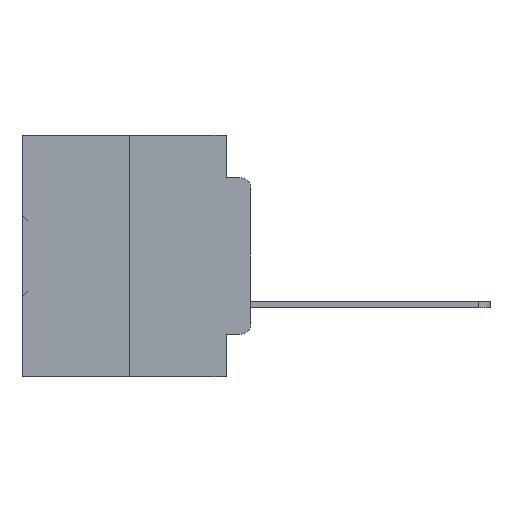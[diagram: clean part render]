
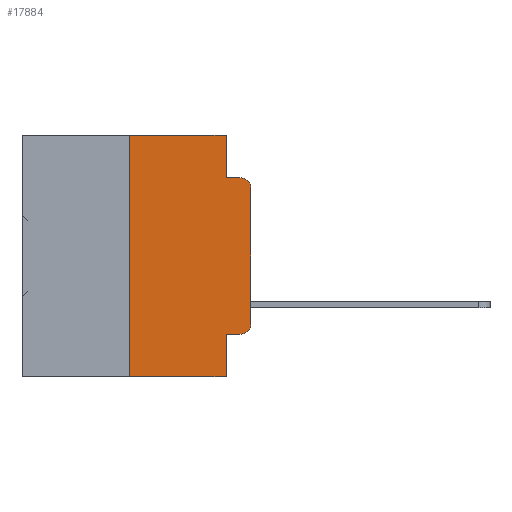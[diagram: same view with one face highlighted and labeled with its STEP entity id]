
A CAD part, left-side view. The second image highlights one B-rep face of the part: STEP entity #17884.
In plain terms, the highlighted planar face has unit normal (-1, 0, 0).
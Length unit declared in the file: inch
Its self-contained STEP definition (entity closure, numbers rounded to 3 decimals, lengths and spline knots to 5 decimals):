
#5 = VERTEX_POINT ( 'NONE', #21967 ) ;
#500 = LINE ( 'NONE', #32016, #10309 ) ;
#594 = DIRECTION ( 'NONE',  ( 0., 0., -1. ) ) ;
#1216 = VERTEX_POINT ( 'NONE', #17893 ) ;
#2350 = DIRECTION ( 'NONE',  ( 0., 0., 1. ) ) ;
#2479 = CARTESIAN_POINT ( 'NONE',  ( 0., 0., 0. ) ) ;
#2881 = VERTEX_POINT ( 'NONE', #8813 ) ;
#3115 = CARTESIAN_POINT ( 'NONE',  ( 0., 0.051, -0.4115 ) ) ;
#3571 = EDGE_CURVE ( 'NONE', #1216, #13545, #20592, .T. ) ;
#4663 = VERTEX_POINT ( 'NONE', #7876 ) ;
#5486 = ORIENTED_EDGE ( 'NONE', *, *, #15837, .T. ) ;
#6073 = VERTEX_POINT ( 'NONE', #37054 ) ;
#7161 = DIRECTION ( 'NONE',  ( 0., -1., 0. ) ) ;
#7540 = VECTOR ( 'NONE', #7161, 39.37008 ) ;
#7876 = CARTESIAN_POINT ( 'NONE',  ( 0., 0.051, -0.4115 ) ) ;
#8208 = DIRECTION ( 'NONE',  ( -1., 0., 0. ) ) ;
#8439 = DIRECTION ( 'NONE',  ( 0., 0., -1. ) ) ;
#8753 = VECTOR ( 'NONE', #594, 39.37008 ) ;
#8813 = CARTESIAN_POINT ( 'NONE',  ( 0., 0., -0.1085 ) ) ;
#8851 = CARTESIAN_POINT ( 'NONE',  ( 0., 0.02, -0.0885 ) ) ;
#8974 = DIRECTION ( 'NONE',  ( 0., -1., 0. ) ) ;
#9942 = VERTEX_POINT ( 'NONE', #20865 ) ;
#10309 = VECTOR ( 'NONE', #2350, 39.37008 ) ;
#10937 = EDGE_CURVE ( 'NONE', #20522, #1216, #16654, .T. ) ;
#11811 = VECTOR ( 'NONE', #24038, 39.37008 ) ;
#11969 = CIRCLE ( 'NONE', #26643, 0.02 ) ;
#13545 = VERTEX_POINT ( 'NONE', #8851 ) ;
#13551 = ORIENTED_EDGE ( 'NONE', *, *, #27134, .T. ) ;
#13850 = VERTEX_POINT ( 'NONE', #27677 ) ;
#15076 = CARTESIAN_POINT ( 'NONE',  ( 0., 0.051, 0. ) ) ;
#15723 = FACE_OUTER_BOUND ( 'NONE', #20264, .T. ) ;
#15837 = EDGE_CURVE ( 'NONE', #2881, #13545, #23999, .T. ) ;
#16018 = EDGE_CURVE ( 'NONE', #4663, #13850, #22566, .T. ) ;
#16654 = LINE ( 'NONE', #15076, #8753 ) ;
#17280 = DIRECTION ( 'NONE',  ( 0., 0., -1. ) ) ;
#17533 = LINE ( 'NONE', #26480, #19832 ) ;
#17884 = ADVANCED_FACE ( 'NONE', ( #15723 ), #35741, .F. ) ;
#17893 = CARTESIAN_POINT ( 'NONE',  ( 0., 0.051, -0.0885 ) ) ;
#19577 = ORIENTED_EDGE ( 'NONE', *, *, #16018, .T. ) ;
#19580 = VECTOR ( 'NONE', #20387, 39.37008 ) ;
#19832 = VECTOR ( 'NONE', #38354, 39.37008 ) ;
#19879 = CARTESIAN_POINT ( 'NONE',  ( 0., 0.02, -0.1085 ) ) ;
#20264 = EDGE_LOOP ( 'NONE', ( #27357, #5486, #26753, #24312, #37018, #27078, #20570, #24830, #19577, #13551 ) ) ;
#20350 = VECTOR ( 'NONE', #8439, 39.37008 ) ;
#20387 = DIRECTION ( 'NONE',  ( 0., 0., 1. ) ) ;
#20522 = VERTEX_POINT ( 'NONE', #36520 ) ;
#20570 = ORIENTED_EDGE ( 'NONE', *, *, #32765, .T. ) ;
#20592 = LINE ( 'NONE', #26526, #11811 ) ;
#20865 = CARTESIAN_POINT ( 'NONE',  ( 0., 0., -0.3915 ) ) ;
#21633 = VECTOR ( 'NONE', #8974, 39.37008 ) ;
#21931 = EDGE_CURVE ( 'NONE', #9942, #2881, #30766, .T. ) ;
#21935 = DIRECTION ( 'NONE',  ( -1., 0., 0. ) ) ;
#21967 = CARTESIAN_POINT ( 'NONE',  ( 0., 0.25, -0.5 ) ) ;
#22069 = CARTESIAN_POINT ( 'NONE',  ( 0., 0.02, -0.3915 ) ) ;
#22077 = CARTESIAN_POINT ( 'NONE',  ( 0., 0.473, 0. ) ) ;
#22566 = LINE ( 'NONE', #3115, #21633 ) ;
#23635 = CARTESIAN_POINT ( 'NONE',  ( 0., 0.473, 0. ) ) ;
#23999 = CIRCLE ( 'NONE', #29081, 0.02 ) ;
#24038 = DIRECTION ( 'NONE',  ( 0., -1., 0. ) ) ;
#24096 = LINE ( 'NONE', #26217, #20350 ) ;
#24312 = ORIENTED_EDGE ( 'NONE', *, *, #10937, .F. ) ;
#24375 = EDGE_CURVE ( 'NONE', #5, #33900, #500, .T. ) ;
#24830 = ORIENTED_EDGE ( 'NONE', *, *, #26684, .F. ) ;
#25496 = CARTESIAN_POINT ( 'NONE',  ( 0., 0.25, 0. ) ) ;
#26217 = CARTESIAN_POINT ( 'NONE',  ( 0., 0.051, 0. ) ) ;
#26480 = CARTESIAN_POINT ( 'NONE',  ( 0., 0.473, -0.5 ) ) ;
#26526 = CARTESIAN_POINT ( 'NONE',  ( 0., 0.051, -0.0885 ) ) ;
#26643 = AXIS2_PLACEMENT_3D ( 'NONE', #22069, #21935, #34331 ) ;
#26684 = EDGE_CURVE ( 'NONE', #4663, #6073, #24096, .T. ) ;
#26753 = ORIENTED_EDGE ( 'NONE', *, *, #3571, .F. ) ;
#27078 = ORIENTED_EDGE ( 'NONE', *, *, #24375, .F. ) ;
#27134 = EDGE_CURVE ( 'NONE', #13850, #9942, #11969, .T. ) ;
#27357 = ORIENTED_EDGE ( 'NONE', *, *, #21931, .T. ) ;
#27677 = CARTESIAN_POINT ( 'NONE',  ( 0., 0.02, -0.4115 ) ) ;
#29081 = AXIS2_PLACEMENT_3D ( 'NONE', #19879, #8208, #17280 ) ;
#29230 = DIRECTION ( 'NONE',  ( 1., 0., 0. ) ) ;
#29871 = AXIS2_PLACEMENT_3D ( 'NONE', #23635, #29230, #32252 ) ;
#30766 = LINE ( 'NONE', #2479, #19580 ) ;
#30790 = LINE ( 'NONE', #22077, #7540 ) ;
#32016 = CARTESIAN_POINT ( 'NONE',  ( 0., 0.25, 0. ) ) ;
#32252 = DIRECTION ( 'NONE',  ( 0., 0., -1. ) ) ;
#32765 = EDGE_CURVE ( 'NONE', #5, #6073, #17533, .T. ) ;
#33900 = VERTEX_POINT ( 'NONE', #25496 ) ;
#34331 = DIRECTION ( 'NONE',  ( 0., 0., -1. ) ) ;
#35741 = PLANE ( 'NONE',  #29871 ) ;
#36520 = CARTESIAN_POINT ( 'NONE',  ( 0., 0.051, 0. ) ) ;
#36851 = EDGE_CURVE ( 'NONE', #33900, #20522, #30790, .T. ) ;
#37018 = ORIENTED_EDGE ( 'NONE', *, *, #36851, .F. ) ;
#37054 = CARTESIAN_POINT ( 'NONE',  ( 0., 0.051, -0.5 ) ) ;
#38354 = DIRECTION ( 'NONE',  ( 0., -1., 0. ) ) ;
